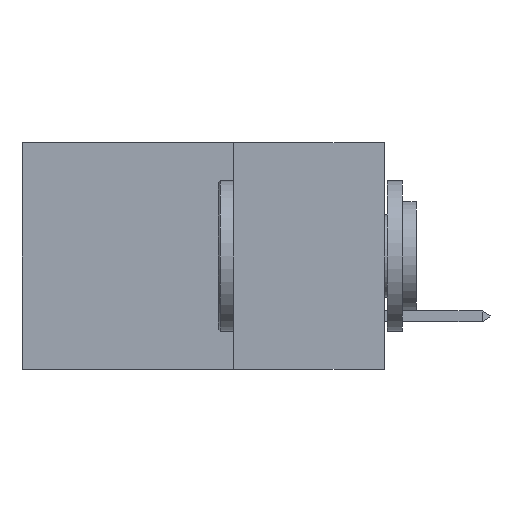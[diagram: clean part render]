
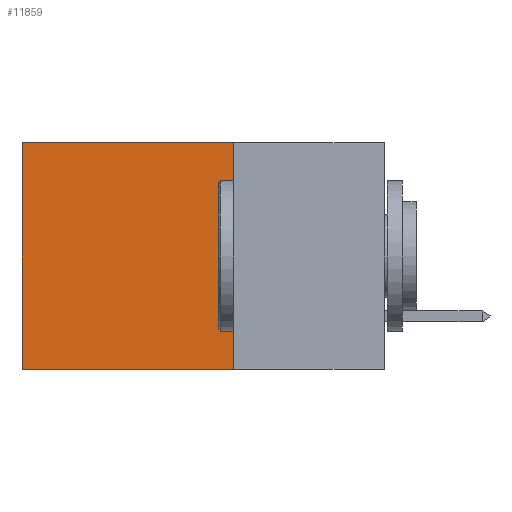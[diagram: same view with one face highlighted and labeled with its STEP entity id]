
A CAD part, left-side view. The second image highlights one B-rep face of the part: STEP entity #11859.
In plain terms, the highlighted planar face has unit normal (-1, 0, 0).
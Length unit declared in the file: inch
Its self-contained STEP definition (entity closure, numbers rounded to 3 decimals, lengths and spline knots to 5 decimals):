
#743 = EDGE_CURVE ( 'NONE', #8101, #10842, #3705, .T. ) ;
#1229 = EDGE_LOOP ( 'NONE', ( #15187, #8939, #14742, #6217 ) ) ;
#1905 = DIRECTION ( 'NONE',  ( 0., 1., 0. ) ) ;
#2910 = CARTESIAN_POINT ( 'NONE',  ( 0.2875, 0.25, 0. ) ) ;
#3445 = PLANE ( 'NONE',  #13107 ) ;
#3705 = LINE ( 'NONE', #8228, #14095 ) ;
#4638 = FACE_OUTER_BOUND ( 'NONE', #1229, .T. ) ;
#4716 = LINE ( 'NONE', #7516, #9905 ) ;
#5223 = DIRECTION ( 'NONE',  ( 0., 0., -1. ) ) ;
#5360 = CARTESIAN_POINT ( 'NONE',  ( 0.2875, 0.6, -0.375 ) ) ;
#5832 = EDGE_CURVE ( 'NONE', #12937, #8260, #12884, .T. ) ;
#5966 = DIRECTION ( 'NONE',  ( 0., 0., -1. ) ) ;
#6217 = ORIENTED_EDGE ( 'NONE', *, *, #5832, .T. ) ;
#7516 = CARTESIAN_POINT ( 'NONE',  ( 0.2875, 0.6, -0.375 ) ) ;
#8101 = VERTEX_POINT ( 'NONE', #11501 ) ;
#8169 = CARTESIAN_POINT ( 'NONE',  ( 0.2875, 0.25, 0. ) ) ;
#8228 = CARTESIAN_POINT ( 'NONE',  ( 0.2875, 0.25, -0.375 ) ) ;
#8260 = VERTEX_POINT ( 'NONE', #10374 ) ;
#8342 = EDGE_CURVE ( 'NONE', #12937, #8101, #15839, .T. ) ;
#8436 = CARTESIAN_POINT ( 'NONE',  ( 0.2875, 0.25, -0.375 ) ) ;
#8939 = ORIENTED_EDGE ( 'NONE', *, *, #743, .F. ) ;
#9183 = EDGE_CURVE ( 'NONE', #8260, #10842, #4716, .T. ) ;
#9615 = VECTOR ( 'NONE', #13794, 39.37008 ) ;
#9905 = VECTOR ( 'NONE', #5223, 39.37008 ) ;
#10374 = CARTESIAN_POINT ( 'NONE',  ( 0.2875, 0.6, 0. ) ) ;
#10842 = VERTEX_POINT ( 'NONE', #5360 ) ;
#11501 = CARTESIAN_POINT ( 'NONE',  ( 0.2875, 0.25, -0.375 ) ) ;
#11856 = DIRECTION ( 'NONE',  ( 0., 0., -1. ) ) ;
#11859 = ADVANCED_FACE ( 'NONE', ( #4638 ), #3445, .F. ) ;
#12884 = LINE ( 'NONE', #2910, #9615 ) ;
#12937 = VERTEX_POINT ( 'NONE', #8169 ) ;
#13107 = AXIS2_PLACEMENT_3D ( 'NONE', #8436, #13261, #5966 ) ;
#13261 = DIRECTION ( 'NONE',  ( 1., 0., 0. ) ) ;
#13794 = DIRECTION ( 'NONE',  ( 0., 1., 0. ) ) ;
#14095 = VECTOR ( 'NONE', #1905, 39.37008 ) ;
#14294 = CARTESIAN_POINT ( 'NONE',  ( 0.2875, 0.25, -0.375 ) ) ;
#14742 = ORIENTED_EDGE ( 'NONE', *, *, #8342, .F. ) ;
#15187 = ORIENTED_EDGE ( 'NONE', *, *, #9183, .T. ) ;
#15462 = VECTOR ( 'NONE', #11856, 39.37008 ) ;
#15839 = LINE ( 'NONE', #14294, #15462 ) ;
